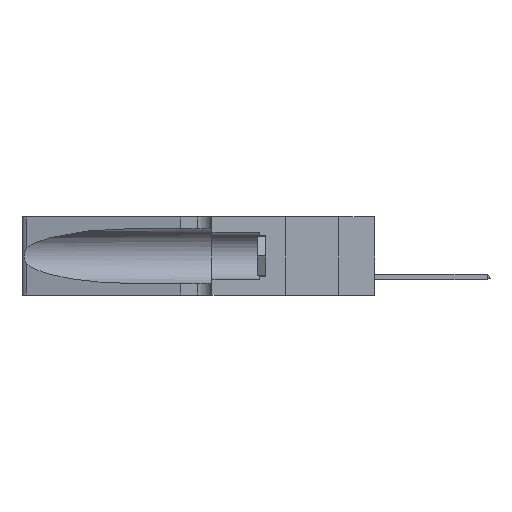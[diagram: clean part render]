
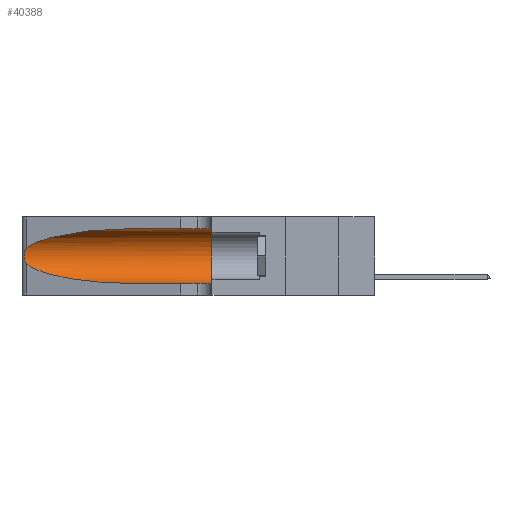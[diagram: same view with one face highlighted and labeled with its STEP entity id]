
A CAD part, left-side view. The second image highlights one B-rep face of the part: STEP entity #40388.
In plain terms, the highlighted cylindrical face has radius 3.308 mm (diameter 6.617 mm), a partial arc.
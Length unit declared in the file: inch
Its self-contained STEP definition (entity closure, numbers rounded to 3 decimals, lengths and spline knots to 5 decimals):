
#1012 = CARTESIAN_POINT ( 'NONE',  ( 0.25487, 1.22718, 0.14631 ) ) ;
#1192 = VECTOR ( 'NONE', #31788, 39.37008 ) ;
#2794 = ORIENTED_EDGE ( 'NONE', *, *, #23438, .T. ) ;
#4208 = CARTESIAN_POINT ( 'NONE',  ( 0.18966, 0.96281, 0.05475 ) ) ;
#4954 = CARTESIAN_POINT ( 'NONE',  ( 0.1305, 1.61858, 0.31525 ) ) ;
#5733 = VERTEX_POINT ( 'NONE', #38325 ) ;
#6917 = CARTESIAN_POINT ( 'NONE',  ( 0.1305, 0.72297, 0.05475 ) ) ;
#7249 = CARTESIAN_POINT ( 'NONE',  ( 0.25854, 1.2359, 0.20912 ) ) ;
#7396 = CARTESIAN_POINT ( 'NONE',  ( 0.26075, 1.23896, 0.19203 ) ) ;
#10448 = CARTESIAN_POINT ( 'NONE',  ( 0.1305, 0.72297, 0.31525 ) ) ;
#10684 = CARTESIAN_POINT ( 'NONE',  ( 0.25787, 1.23484, 0.2124 ) ) ;
#11118 = DIRECTION ( 'NONE',  ( 0., 0., -1. ) ) ;
#11324 = ORIENTED_EDGE ( 'NONE', *, *, #34331, .T. ) ;
#11553 = FACE_OUTER_BOUND ( 'NONE', #21218, .T. ) ;
#14004 = ORIENTED_EDGE ( 'NONE', *, *, #41853, .T. ) ;
#14100 = VERTEX_POINT ( 'NONE', #23969 ) ;
#15929 = CIRCLE ( 'NONE', #39394, 0.13025 ) ;
#16660 = VECTOR ( 'NONE', #26615, 39.37008 ) ;
#17637 = CARTESIAN_POINT ( 'NONE',  ( 0.25789, 1.23486, 0.15765 ) ) ;
#19687 = CARTESIAN_POINT ( 'NONE',  ( 0.25487, 1.22718, 0.14631 ) ) ;
#21218 = EDGE_LOOP ( 'NONE', ( #2794, #25360, #11324, #14004, #38097, #37420 ) ) ;
#21435 = VERTEX_POINT ( 'NONE', #19687 ) ;
#23438 = EDGE_CURVE ( 'NONE', #29795, #42147, #38854, .T. ) ;
#23792 = CARTESIAN_POINT ( 'NONE',  ( 0.2373, 1.15595, 0.28018 ) ) ;
#23963 = CARTESIAN_POINT ( 'NONE',  ( 0.2373, 1.15595, 0.08982 ) ) ;
#23969 = CARTESIAN_POINT ( 'NONE',  ( 0.1305, 0.35, 0.31525 ) ) ;
#25360 = ORIENTED_EDGE ( 'NONE', *, *, #35525, .T. ) ;
#26021 = CARTESIAN_POINT ( 'NONE',  ( 0.1305, 0.35, 0.185 ) ) ;
#26351 = CARTESIAN_POINT ( 'NONE',  ( 0.1305, 1.61858, 0.05475 ) ) ;
#26615 = DIRECTION ( 'NONE',  ( 0., -1., 0. ) ) ;
#27187 = CARTESIAN_POINT ( 'NONE',  ( 0.26018, 1.23835, 0.19895 ) ) ;
#28268 = EDGE_CURVE ( 'NONE', #29795, #14100, #42389, .T. ) ;
#29795 = VERTEX_POINT ( 'NONE', #30614 ) ;
#30266 = EDGE_CURVE ( 'NONE', #14100, #5733, #15929, .T. ) ;
#30614 = CARTESIAN_POINT ( 'NONE',  ( 0.1305, 0.72297, 0.31525 ) ) ;
#30642 = CARTESIAN_POINT ( 'NONE',  ( 0.25487, 1.22718, 0.22369 ) ) ;
#30797 = CARTESIAN_POINT ( 'NONE',  ( 0.25639, 1.23186, 0.15144 ) ) ;
#30913 = CARTESIAN_POINT ( 'NONE',  ( 0.1305, 1.61858, 0.185 ) ) ;
#31226 =( BOUNDED_CURVE ( )  B_SPLINE_CURVE ( 3, ( #33307, #23963, #4208, #6917 ),
 .UNSPECIFIED., .F., .F. ) 
 B_SPLINE_CURVE_WITH_KNOTS ( ( 4, 4 ),
 ( 3.44316, 4.71239 ),
 .UNSPECIFIED. ) 
 CURVE ( )  GEOMETRIC_REPRESENTATION_ITEM ( )  RATIONAL_B_SPLINE_CURVE ( ( 1., 0.87, 0.87, 1. ) ) 
 REPRESENTATION_ITEM ( '' )  );
#31788 = DIRECTION ( 'NONE',  ( 0., -1., 0. ) ) ;
#32630 = CARTESIAN_POINT ( 'NONE',  ( 0.1305, 0.72297, 0.05475 ) ) ;
#33307 = CARTESIAN_POINT ( 'NONE',  ( 0.25487, 1.22718, 0.14631 ) ) ;
#33643 = CARTESIAN_POINT ( 'NONE',  ( 0.25639, 1.23184, 0.21858 ) ) ;
#33787 = CARTESIAN_POINT ( 'NONE',  ( 0.25555, 1.22993, 0.14849 ) ) ;
#34095 = CARTESIAN_POINT ( 'NONE',  ( 0.25856, 1.23593, 0.16098 ) ) ;
#34331 = EDGE_CURVE ( 'NONE', #21435, #42538, #31226, .T. ) ;
#35525 = EDGE_CURVE ( 'NONE', #42147, #21435, #35705, .T. ) ;
#35705 = B_SPLINE_CURVE_WITH_KNOTS ( 'NONE', 3,
 ( #30642, #40521, #33643, #10684, #7249, #27187, #7396, #40370, #37379, #34095, #17637, #30797, #33787, #1012 ),
 .UNSPECIFIED., .F., .F.,
 ( 4, 2, 2, 2, 2, 2, 4 ),
 ( 0., 0.00027, 0.00053, 0.00107, 0.0016, 0.00187, 0.00214 ),
 .UNSPECIFIED. ) ;
#36095 = AXIS2_PLACEMENT_3D ( 'NONE', #30913, #37492, #11118 ) ;
#36699 = CARTESIAN_POINT ( 'NONE',  ( 0.18966, 0.96281, 0.31525 ) ) ;
#37379 = CARTESIAN_POINT ( 'NONE',  ( 0.26017, 1.23833, 0.17102 ) ) ;
#37420 = ORIENTED_EDGE ( 'NONE', *, *, #28268, .F. ) ;
#37492 = DIRECTION ( 'NONE',  ( 0., -1., 0. ) ) ;
#38097 = ORIENTED_EDGE ( 'NONE', *, *, #30266, .F. ) ;
#38325 = CARTESIAN_POINT ( 'NONE',  ( 0.1305, 0.35, 0.05475 ) ) ;
#38854 =( BOUNDED_CURVE ( )  B_SPLINE_CURVE ( 3, ( #10448, #36699, #23792, #40424 ),
 .UNSPECIFIED., .F., .F. ) 
 B_SPLINE_CURVE_WITH_KNOTS ( ( 4, 4 ),
 ( 1.5708, 2.84003 ),
 .UNSPECIFIED. ) 
 CURVE ( )  GEOMETRIC_REPRESENTATION_ITEM ( )  RATIONAL_B_SPLINE_CURVE ( ( 1., 0.87, 0.87, 1. ) ) 
 REPRESENTATION_ITEM ( '' )  );
#39394 = AXIS2_PLACEMENT_3D ( 'NONE', #26021, #42233, #42505 ) ;
#39406 = CYLINDRICAL_SURFACE ( 'NONE', #36095, 0.13025 ) ;
#40370 = CARTESIAN_POINT ( 'NONE',  ( 0.26075, 1.23896, 0.178 ) ) ;
#40388 = ADVANCED_FACE ( 'NONE', ( #11553 ), #39406, .F. ) ;
#40424 = CARTESIAN_POINT ( 'NONE',  ( 0.25487, 1.22718, 0.22369 ) ) ;
#40521 = CARTESIAN_POINT ( 'NONE',  ( 0.25555, 1.22994, 0.2215 ) ) ;
#41276 = CARTESIAN_POINT ( 'NONE',  ( 0.25487, 1.22718, 0.22369 ) ) ;
#41853 = EDGE_CURVE ( 'NONE', #42538, #5733, #42419, .T. ) ;
#42147 = VERTEX_POINT ( 'NONE', #41276 ) ;
#42233 = DIRECTION ( 'NONE',  ( 0., 1., 0. ) ) ;
#42389 = LINE ( 'NONE', #4954, #1192 ) ;
#42419 = LINE ( 'NONE', #26351, #16660 ) ;
#42505 = DIRECTION ( 'NONE',  ( 0., 0., 1. ) ) ;
#42538 = VERTEX_POINT ( 'NONE', #32630 ) ;
